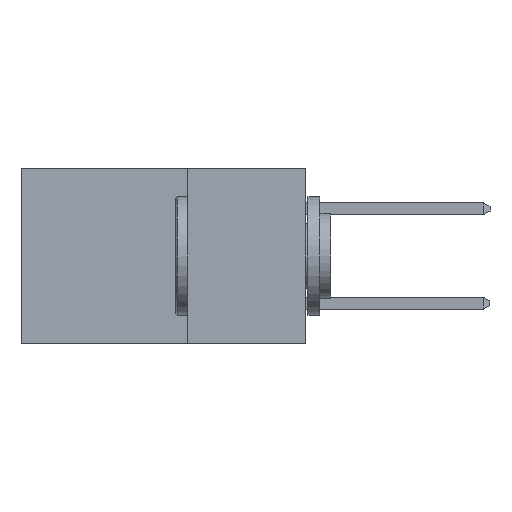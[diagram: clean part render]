
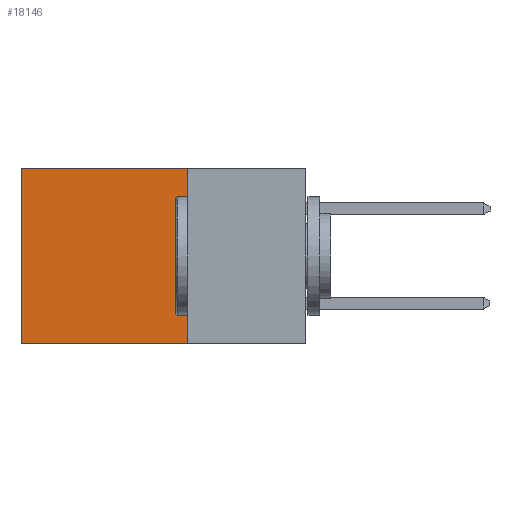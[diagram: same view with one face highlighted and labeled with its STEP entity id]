
A CAD part, left-side view. The second image highlights one B-rep face of the part: STEP entity #18146.
In plain terms, the highlighted planar face has unit normal (-1, 0, 0).
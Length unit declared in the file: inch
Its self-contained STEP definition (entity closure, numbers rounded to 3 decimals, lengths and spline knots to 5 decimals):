
#669 = VERTEX_POINT ( 'NONE', #2692 ) ;
#1073 = CARTESIAN_POINT ( 'NONE',  ( 0.298, 0.25, 0. ) ) ;
#1308 = AXIS2_PLACEMENT_3D ( 'NONE', #7049, #19531, #10222 ) ;
#1310 = EDGE_CURVE ( 'NONE', #13310, #1965, #13242, .T. ) ;
#1965 = VERTEX_POINT ( 'NONE', #7137 ) ;
#2427 = ORIENTED_EDGE ( 'NONE', *, *, #17199, .F. ) ;
#2683 = DIRECTION ( 'NONE',  ( 0., 1., 0. ) ) ;
#2692 = CARTESIAN_POINT ( 'NONE',  ( 0.298, 0.25, 0. ) ) ;
#5491 = PLANE ( 'NONE',  #1308 ) ;
#6154 = CARTESIAN_POINT ( 'NONE',  ( 0.298, 0.6, 0. ) ) ;
#6666 = ORIENTED_EDGE ( 'NONE', *, *, #8949, .T. ) ;
#7049 = CARTESIAN_POINT ( 'NONE',  ( 0.298, 0.25, 0. ) ) ;
#7137 = CARTESIAN_POINT ( 'NONE',  ( 0.298, 0.6, -0.37 ) ) ;
#7690 = VECTOR ( 'NONE', #10478, 39.37008 ) ;
#8225 = CARTESIAN_POINT ( 'NONE',  ( 0.298, 0.25, -0.37 ) ) ;
#8275 = CARTESIAN_POINT ( 'NONE',  ( 0.298, 0.6, 0. ) ) ;
#8330 = VECTOR ( 'NONE', #15309, 39.37008 ) ;
#8933 = CARTESIAN_POINT ( 'NONE',  ( 0.298, 0.25, 0. ) ) ;
#8949 = EDGE_CURVE ( 'NONE', #669, #13310, #16501, .T. ) ;
#9103 = ORIENTED_EDGE ( 'NONE', *, *, #1310, .T. ) ;
#9156 = CARTESIAN_POINT ( 'NONE',  ( 0.298, 0.25, -0.37 ) ) ;
#10222 = DIRECTION ( 'NONE',  ( 0., 0., -1. ) ) ;
#10387 = EDGE_LOOP ( 'NONE', ( #9103, #13146, #2427, #6666 ) ) ;
#10478 = DIRECTION ( 'NONE',  ( 0., 0., -1. ) ) ;
#12469 = LINE ( 'NONE', #9156, #8330 ) ;
#12819 = VECTOR ( 'NONE', #2683, 39.37008 ) ;
#13146 = ORIENTED_EDGE ( 'NONE', *, *, #14631, .F. ) ;
#13242 = LINE ( 'NONE', #8275, #17400 ) ;
#13310 = VERTEX_POINT ( 'NONE', #6154 ) ;
#13378 = DIRECTION ( 'NONE',  ( 0., 0., -1. ) ) ;
#14315 = FACE_OUTER_BOUND ( 'NONE', #10387, .T. ) ;
#14631 = EDGE_CURVE ( 'NONE', #18692, #1965, #12469, .T. ) ;
#15309 = DIRECTION ( 'NONE',  ( 0., 1., 0. ) ) ;
#16501 = LINE ( 'NONE', #1073, #12819 ) ;
#17199 = EDGE_CURVE ( 'NONE', #669, #18692, #19625, .T. ) ;
#17400 = VECTOR ( 'NONE', #13378, 39.37008 ) ;
#18146 = ADVANCED_FACE ( 'NONE', ( #14315 ), #5491, .F. ) ;
#18692 = VERTEX_POINT ( 'NONE', #8225 ) ;
#19531 = DIRECTION ( 'NONE',  ( 1., 0., 0. ) ) ;
#19625 = LINE ( 'NONE', #8933, #7690 ) ;
